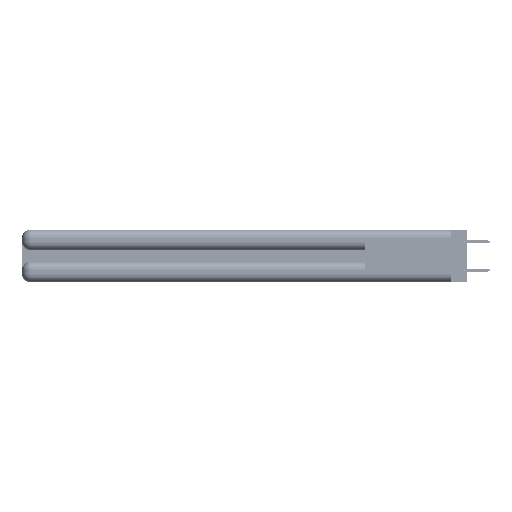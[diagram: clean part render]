
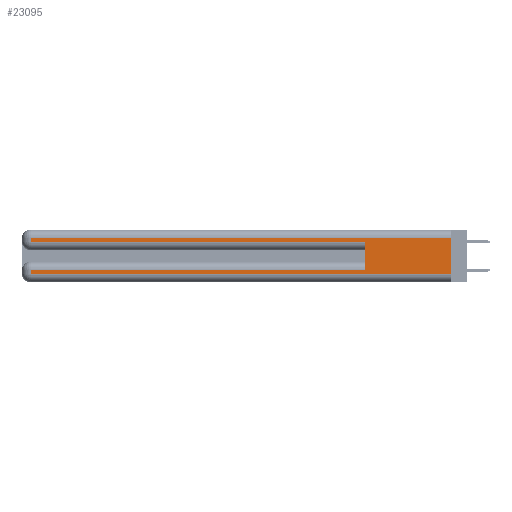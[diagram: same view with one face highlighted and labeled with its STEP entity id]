
A CAD part, left-side view. The second image highlights one B-rep face of the part: STEP entity #23095.
In plain terms, the highlighted planar face has unit normal (-1, 0, 0).
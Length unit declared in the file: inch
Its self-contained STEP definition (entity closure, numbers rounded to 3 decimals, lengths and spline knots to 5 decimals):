
#219 = CARTESIAN_POINT ( 'NONE',  ( 0., 2.94, 0.06 ) ) ;
#305 = VECTOR ( 'NONE', #24402, 39.37008 ) ;
#1232 = CARTESIAN_POINT ( 'NONE',  ( 0., 2.94, 0.085 ) ) ;
#1502 = FACE_OUTER_BOUND ( 'NONE', #45738, .T. ) ;
#2092 = VERTEX_POINT ( 'NONE', #50758 ) ;
#2248 = VECTOR ( 'NONE', #46938, 39.37008 ) ;
#4875 = CARTESIAN_POINT ( 'NONE',  ( 0., 0.6, 0.145 ) ) ;
#6347 = EDGE_CURVE ( 'NONE', #26838, #8749, #49909, .T. ) ;
#6669 = EDGE_CURVE ( 'NONE', #6738, #8749, #41218, .T. ) ;
#6738 = VERTEX_POINT ( 'NONE', #51813 ) ;
#6950 = CARTESIAN_POINT ( 'NONE',  ( 0., 2.94, 0.37 ) ) ;
#7486 = EDGE_CURVE ( 'NONE', #28683, #2092, #35198, .T. ) ;
#8206 = DIRECTION ( 'NONE',  ( 0., 0., -1. ) ) ;
#8749 = VERTEX_POINT ( 'NONE', #45405 ) ;
#11381 = DIRECTION ( 'NONE',  ( 0., 0., -1. ) ) ;
#11398 = CARTESIAN_POINT ( 'NONE',  ( 0., 0., 0.285 ) ) ;
#12106 = ORIENTED_EDGE ( 'NONE', *, *, #22897, .T. ) ;
#12703 = CARTESIAN_POINT ( 'NONE',  ( 0., 0., 0.06 ) ) ;
#12717 = DIRECTION ( 'NONE',  ( 0., 0., -1. ) ) ;
#12912 = LINE ( 'NONE', #24221, #305 ) ;
#13979 = ORIENTED_EDGE ( 'NONE', *, *, #25077, .T. ) ;
#15290 = VECTOR ( 'NONE', #17450, 39.37008 ) ;
#16325 = VECTOR ( 'NONE', #45129, 39.37008 ) ;
#16606 = LINE ( 'NONE', #42886, #15290 ) ;
#17093 = CARTESIAN_POINT ( 'NONE',  ( 0., 2.94, 0.31 ) ) ;
#17450 = DIRECTION ( 'NONE',  ( 0., 0., -1. ) ) ;
#21135 = EDGE_CURVE ( 'NONE', #31700, #2092, #29508, .T. ) ;
#21178 = DIRECTION ( 'NONE',  ( 0., -1., 0. ) ) ;
#22040 = LINE ( 'NONE', #6950, #54288 ) ;
#22081 = LINE ( 'NONE', #42740, #2248 ) ;
#22245 = AXIS2_PLACEMENT_3D ( 'NONE', #29248, #33536, #8206 ) ;
#22704 = ORIENTED_EDGE ( 'NONE', *, *, #37895, .T. ) ;
#22897 = EDGE_CURVE ( 'NONE', #51622, #31700, #22040, .T. ) ;
#23095 = ADVANCED_FACE ( 'NONE', ( #1502 ), #54422, .F. ) ;
#24221 = CARTESIAN_POINT ( 'NONE',  ( 0., 0., 0.085 ) ) ;
#24402 = DIRECTION ( 'NONE',  ( 0., 1., 0. ) ) ;
#25077 = EDGE_CURVE ( 'NONE', #36771, #26838, #16606, .T. ) ;
#26838 = VERTEX_POINT ( 'NONE', #53342 ) ;
#27969 = CARTESIAN_POINT ( 'NONE',  ( 0., 0., 0.31 ) ) ;
#28683 = VERTEX_POINT ( 'NONE', #27969 ) ;
#29248 = CARTESIAN_POINT ( 'NONE',  ( 0., 0., 0.37 ) ) ;
#29508 = LINE ( 'NONE', #12703, #50534 ) ;
#31700 = VERTEX_POINT ( 'NONE', #219 ) ;
#33536 = DIRECTION ( 'NONE',  ( 1., 0., 0. ) ) ;
#33783 = CARTESIAN_POINT ( 'NONE',  ( 0., 0., 0.37 ) ) ;
#35198 = LINE ( 'NONE', #33783, #45042 ) ;
#36771 = VERTEX_POINT ( 'NONE', #17093 ) ;
#37895 = EDGE_CURVE ( 'NONE', #28683, #36771, #22081, .T. ) ;
#39875 = VECTOR ( 'NONE', #42891, 39.37008 ) ;
#41218 = LINE ( 'NONE', #4875, #39875 ) ;
#42710 = EDGE_CURVE ( 'NONE', #6738, #51622, #12912, .T. ) ;
#42740 = CARTESIAN_POINT ( 'NONE',  ( 0., 0., 0.31 ) ) ;
#42886 = CARTESIAN_POINT ( 'NONE',  ( 0., 2.94, 0.37 ) ) ;
#42891 = DIRECTION ( 'NONE',  ( 0., 0., 1. ) ) ;
#45042 = VECTOR ( 'NONE', #12717, 39.37008 ) ;
#45093 = ORIENTED_EDGE ( 'NONE', *, *, #6669, .F. ) ;
#45129 = DIRECTION ( 'NONE',  ( 0., -1., 0. ) ) ;
#45347 = ORIENTED_EDGE ( 'NONE', *, *, #42710, .T. ) ;
#45405 = CARTESIAN_POINT ( 'NONE',  ( 0., 0.6, 0.285 ) ) ;
#45738 = EDGE_LOOP ( 'NONE', ( #46244, #22704, #13979, #49660, #45093, #45347, #12106, #47650 ) ) ;
#46244 = ORIENTED_EDGE ( 'NONE', *, *, #7486, .F. ) ;
#46938 = DIRECTION ( 'NONE',  ( 0., 1., 0. ) ) ;
#47650 = ORIENTED_EDGE ( 'NONE', *, *, #21135, .T. ) ;
#49660 = ORIENTED_EDGE ( 'NONE', *, *, #6347, .T. ) ;
#49909 = LINE ( 'NONE', #11398, #16325 ) ;
#50534 = VECTOR ( 'NONE', #21178, 39.37008 ) ;
#50758 = CARTESIAN_POINT ( 'NONE',  ( 0., 0., 0.06 ) ) ;
#51622 = VERTEX_POINT ( 'NONE', #1232 ) ;
#51813 = CARTESIAN_POINT ( 'NONE',  ( 0., 0.6, 0.085 ) ) ;
#53342 = CARTESIAN_POINT ( 'NONE',  ( 0., 2.94, 0.285 ) ) ;
#54288 = VECTOR ( 'NONE', #11381, 39.37008 ) ;
#54422 = PLANE ( 'NONE',  #22245 ) ;
